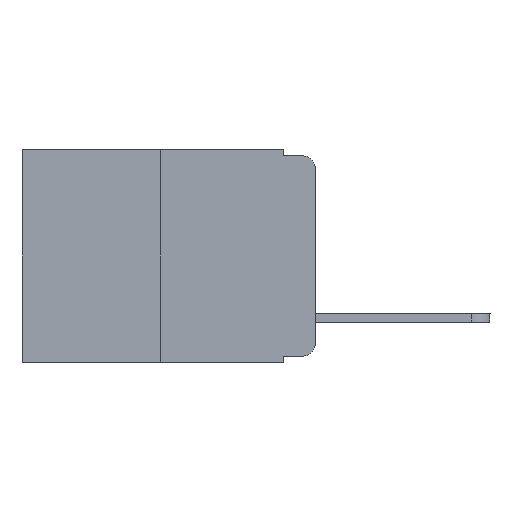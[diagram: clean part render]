
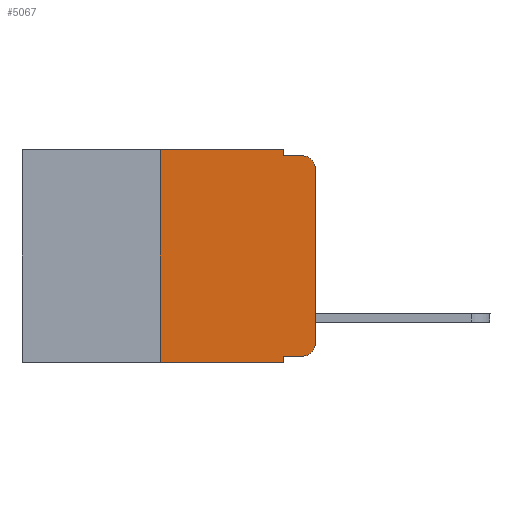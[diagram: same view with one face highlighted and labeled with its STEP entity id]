
A CAD part, left-side view. The second image highlights one B-rep face of the part: STEP entity #5067.
In plain terms, the highlighted planar face has unit normal (-1, 0, 0).
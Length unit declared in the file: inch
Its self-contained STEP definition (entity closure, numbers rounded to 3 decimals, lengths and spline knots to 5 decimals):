
#65 = VERTEX_POINT ( 'NONE', #7313 ) ;
#95 = AXIS2_PLACEMENT_3D ( 'NONE', #3002, #7437, #1988 ) ;
#259 = VERTEX_POINT ( 'NONE', #4006 ) ;
#474 = CARTESIAN_POINT ( 'NONE',  ( 0., 0.051, 0. ) ) ;
#562 = CARTESIAN_POINT ( 'NONE',  ( 0., 0.473, 0. ) ) ;
#632 = EDGE_LOOP ( 'NONE', ( #5985, #1501, #11318, #3693, #6986, #12744, #7680, #937, #10285, #10395 ) ) ;
#678 = VECTOR ( 'NONE', #6696, 39.37008 ) ;
#785 = CIRCLE ( 'NONE', #1963, 0.02 ) ;
#884 = CARTESIAN_POINT ( 'NONE',  ( 0., 0.051, -0.01 ) ) ;
#912 = DIRECTION ( 'NONE',  ( 0., 0., -1. ) ) ;
#937 = ORIENTED_EDGE ( 'NONE', *, *, #5194, .F. ) ;
#974 = DIRECTION ( 'NONE',  ( -1., 0., 0. ) ) ;
#1284 = DIRECTION ( 'NONE',  ( 0., 0., 1. ) ) ;
#1501 = ORIENTED_EDGE ( 'NONE', *, *, #13026, .T. ) ;
#1589 = DIRECTION ( 'NONE',  ( 0., -1., 0. ) ) ;
#1755 = CARTESIAN_POINT ( 'NONE',  ( 0., 0.02, -0.333 ) ) ;
#1963 = AXIS2_PLACEMENT_3D ( 'NONE', #2054, #974, #8419 ) ;
#1988 = DIRECTION ( 'NONE',  ( 0., 0., -1. ) ) ;
#2017 = CIRCLE ( 'NONE', #12893, 0.02 ) ;
#2054 = CARTESIAN_POINT ( 'NONE',  ( 0., 0.02, -0.03 ) ) ;
#2207 = FACE_OUTER_BOUND ( 'NONE', #632, .T. ) ;
#2241 = CARTESIAN_POINT ( 'NONE',  ( 0., 0.25, 0. ) ) ;
#2319 = EDGE_CURVE ( 'NONE', #6729, #7184, #2017, .T. ) ;
#2366 = DIRECTION ( 'NONE',  ( 0., 0., -1. ) ) ;
#2545 = VERTEX_POINT ( 'NONE', #884 ) ;
#2653 = VECTOR ( 'NONE', #9932, 39.37008 ) ;
#2755 = CARTESIAN_POINT ( 'NONE',  ( 0., 0., -0.313 ) ) ;
#2968 = VERTEX_POINT ( 'NONE', #10392 ) ;
#3002 = CARTESIAN_POINT ( 'NONE',  ( 0., 0.473, 0. ) ) ;
#3339 = EDGE_CURVE ( 'NONE', #2545, #3859, #11447, .T. ) ;
#3525 = LINE ( 'NONE', #8143, #12834 ) ;
#3551 = CARTESIAN_POINT ( 'NONE',  ( 0., 0.051, -0.01 ) ) ;
#3693 = ORIENTED_EDGE ( 'NONE', *, *, #3930, .F. ) ;
#3859 = VERTEX_POINT ( 'NONE', #8399 ) ;
#3930 = EDGE_CURVE ( 'NONE', #2968, #2545, #11864, .T. ) ;
#4006 = CARTESIAN_POINT ( 'NONE',  ( 0., 0.051, -0.333 ) ) ;
#4572 = CARTESIAN_POINT ( 'NONE',  ( 0., 0.02, -0.313 ) ) ;
#4816 = VERTEX_POINT ( 'NONE', #13588 ) ;
#4868 = LINE ( 'NONE', #2241, #678 ) ;
#5067 = ADVANCED_FACE ( 'NONE', ( #2207 ), #13819, .F. ) ;
#5194 = EDGE_CURVE ( 'NONE', #259, #65, #6399, .T. ) ;
#5273 = EDGE_CURVE ( 'NONE', #8228, #65, #3525, .T. ) ;
#5976 = LINE ( 'NONE', #562, #12048 ) ;
#5985 = ORIENTED_EDGE ( 'NONE', *, *, #11817, .T. ) ;
#6389 = CARTESIAN_POINT ( 'NONE',  ( 0., 0.051, 0. ) ) ;
#6399 = LINE ( 'NONE', #474, #6552 ) ;
#6552 = VECTOR ( 'NONE', #13464, 39.37008 ) ;
#6696 = DIRECTION ( 'NONE',  ( 0., 0., 1. ) ) ;
#6729 = VERTEX_POINT ( 'NONE', #1755 ) ;
#6771 = CARTESIAN_POINT ( 'NONE',  ( 0., 0., 0. ) ) ;
#6986 = ORIENTED_EDGE ( 'NONE', *, *, #12866, .F. ) ;
#7184 = VERTEX_POINT ( 'NONE', #2755 ) ;
#7313 = CARTESIAN_POINT ( 'NONE',  ( 0., 0.051, -0.343 ) ) ;
#7437 = DIRECTION ( 'NONE',  ( 1., 0., 0. ) ) ;
#7680 = ORIENTED_EDGE ( 'NONE', *, *, #5273, .T. ) ;
#8143 = CARTESIAN_POINT ( 'NONE',  ( 0., 0.473, -0.343 ) ) ;
#8228 = VERTEX_POINT ( 'NONE', #8722 ) ;
#8231 = DIRECTION ( 'NONE',  ( 0., -1., 0. ) ) ;
#8313 = DIRECTION ( 'NONE',  ( 0., -1., 0. ) ) ;
#8399 = CARTESIAN_POINT ( 'NONE',  ( 0., 0.02, -0.01 ) ) ;
#8419 = DIRECTION ( 'NONE',  ( 0., 0., -1. ) ) ;
#8722 = CARTESIAN_POINT ( 'NONE',  ( 0., 0.25, -0.343 ) ) ;
#8823 = DIRECTION ( 'NONE',  ( -1., 0., 0. ) ) ;
#8876 = VERTEX_POINT ( 'NONE', #13044 ) ;
#9660 = LINE ( 'NONE', #13540, #12032 ) ;
#9932 = DIRECTION ( 'NONE',  ( 0., -1., 0. ) ) ;
#10285 = ORIENTED_EDGE ( 'NONE', *, *, #13556, .T. ) ;
#10392 = CARTESIAN_POINT ( 'NONE',  ( 0., 0.051, 0. ) ) ;
#10395 = ORIENTED_EDGE ( 'NONE', *, *, #2319, .T. ) ;
#11150 = EDGE_CURVE ( 'NONE', #8228, #8876, #4868, .T. ) ;
#11318 = ORIENTED_EDGE ( 'NONE', *, *, #3339, .F. ) ;
#11447 = LINE ( 'NONE', #3551, #2653 ) ;
#11817 = EDGE_CURVE ( 'NONE', #7184, #4816, #13431, .T. ) ;
#11864 = LINE ( 'NONE', #6389, #12362 ) ;
#12032 = VECTOR ( 'NONE', #8313, 39.37008 ) ;
#12048 = VECTOR ( 'NONE', #8231, 39.37008 ) ;
#12362 = VECTOR ( 'NONE', #912, 39.37008 ) ;
#12744 = ORIENTED_EDGE ( 'NONE', *, *, #11150, .F. ) ;
#12834 = VECTOR ( 'NONE', #1589, 39.37008 ) ;
#12866 = EDGE_CURVE ( 'NONE', #8876, #2968, #5976, .T. ) ;
#12893 = AXIS2_PLACEMENT_3D ( 'NONE', #4572, #8823, #2366 ) ;
#13026 = EDGE_CURVE ( 'NONE', #4816, #3859, #785, .T. ) ;
#13044 = CARTESIAN_POINT ( 'NONE',  ( 0., 0.25, 0. ) ) ;
#13089 = VECTOR ( 'NONE', #1284, 39.37008 ) ;
#13431 = LINE ( 'NONE', #6771, #13089 ) ;
#13464 = DIRECTION ( 'NONE',  ( 0., 0., -1. ) ) ;
#13540 = CARTESIAN_POINT ( 'NONE',  ( 0., 0.051, -0.333 ) ) ;
#13556 = EDGE_CURVE ( 'NONE', #259, #6729, #9660, .T. ) ;
#13588 = CARTESIAN_POINT ( 'NONE',  ( 0., 0., -0.03 ) ) ;
#13819 = PLANE ( 'NONE',  #95 ) ;
